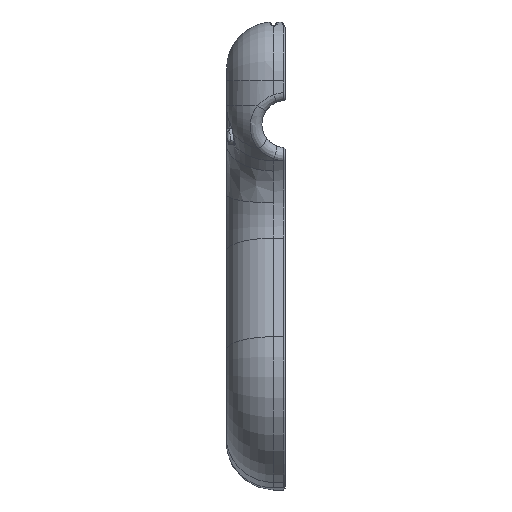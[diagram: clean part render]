
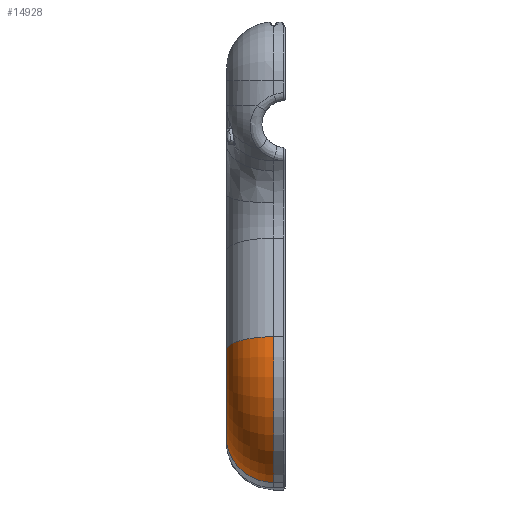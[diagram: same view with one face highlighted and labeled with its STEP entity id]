
A CAD part, left-side view. The second image highlights one B-rep face of the part: STEP entity #14928.
In plain terms, the highlighted toroidal (fillet/blend) face has major radius 18 mm and minor radius 12 mm.
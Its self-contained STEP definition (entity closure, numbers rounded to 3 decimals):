
#3864 = CYLINDRICAL_SURFACE('',#3865,30.);
#3865 = AXIS2_PLACEMENT_3D('',#3866,#3867,#3868);
#3866 = CARTESIAN_POINT('',(-25.893,-15.,-79.431));
#3867 = DIRECTION('',(0.,1.,0.));
#3868 = DIRECTION('',(-0.276,0.,-0.961));
#8954 = VERTEX_POINT('',#8955);
#8955 = CARTESIAN_POINT('',(-34.162,3.,-108.269));
#8992 = CYLINDRICAL_SURFACE('',#8993,12.);
#8993 = AXIS2_PLACEMENT_3D('',#8994,#8995,#8996);
#8994 = CARTESIAN_POINT('',(-26.048,3.,-98.112));
#8995 = DIRECTION('',(-0.961,0.,0.276));
#8996 = DIRECTION('',(-0.276,0.,-0.961));
#9010 = VERTEX_POINT('',#9011);
#9011 = CARTESIAN_POINT('',(-54.731,3.,-71.162));
#9032 = EDGE_CURVE('',#8954,#9010,#9033,.T.);
#9033 = SURFACE_CURVE('',#9034,(#9039,#9046),.PCURVE_S1.);
#9034 = CIRCLE('',#9035,30.);
#9035 = AXIS2_PLACEMENT_3D('',#9036,#9037,#9038);
#9036 = CARTESIAN_POINT('',(-25.893,3.,-79.431));
#9037 = DIRECTION('',(0.,1.,0.));
#9038 = DIRECTION('',(-0.276,0.,-0.961));
#9039 = PCURVE('',#3864,#9040);
#9040 = DEFINITIONAL_REPRESENTATION('',(#9041),#9045);
#9041 = LINE('',#9042,#9043);
#9042 = CARTESIAN_POINT('',(0.,18.));
#9043 = VECTOR('',#9044,1.);
#9044 = DIRECTION('',(1.,0.));
#9045 = ( GEOMETRIC_REPRESENTATION_CONTEXT(2) 
PARAMETRIC_REPRESENTATION_CONTEXT() REPRESENTATION_CONTEXT('2D SPACE',''
  ) );
#9046 = PCURVE('',#9047,#9052);
#9047 = TOROIDAL_SURFACE('',#9048,18.,12.);
#9048 = AXIS2_PLACEMENT_3D('',#9049,#9050,#9051);
#9049 = CARTESIAN_POINT('',(-25.893,3.,-79.431));
#9050 = DIRECTION('',(0.,1.,0.));
#9051 = DIRECTION('',(-0.276,0.,-0.961));
#9052 = DEFINITIONAL_REPRESENTATION('',(#9053),#9057);
#9053 = LINE('',#9054,#9055);
#9054 = CARTESIAN_POINT('',(0.,0.));
#9055 = VECTOR('',#9056,1.);
#9056 = DIRECTION('',(1.,0.));
#9057 = ( GEOMETRIC_REPRESENTATION_CONTEXT(2) 
PARAMETRIC_REPRESENTATION_CONTEXT() REPRESENTATION_CONTEXT('2D SPACE',''
  ) );
#9101 = CYLINDRICAL_SURFACE('',#9102,12.);
#9102 = AXIS2_PLACEMENT_3D('',#9103,#9104,#9105);
#9103 = CARTESIAN_POINT('',(-43.196,3.,-74.47));
#9104 = DIRECTION('',(0.276,0.,0.961));
#9105 = DIRECTION('',(-0.961,0.,0.276));
#14800 = PLANE('',#14801);
#14801 = AXIS2_PLACEMENT_3D('',#14802,#14803,#14804);
#14802 = CARTESIAN_POINT('',(10.936,15.,-32.273));
#14803 = DIRECTION('',(0.,1.,0.));
#14804 = DIRECTION('',(0.,0.,1.));
#14886 = VERTEX_POINT('',#14887);
#14887 = CARTESIAN_POINT('',(-30.855,15.,-96.734));
#14908 = EDGE_CURVE('',#8954,#14886,#14909,.T.);
#14909 = SURFACE_CURVE('',#14910,(#14915,#14921),.PCURVE_S1.);
#14910 = CIRCLE('',#14911,12.);
#14911 = AXIS2_PLACEMENT_3D('',#14912,#14913,#14914);
#14912 = CARTESIAN_POINT('',(-30.855,3.,-96.734));
#14913 = DIRECTION('',(0.961,0.,-0.276));
#14914 = DIRECTION('',(-0.276,0.,-0.961));
#14915 = PCURVE('',#8992,#14916);
#14916 = DEFINITIONAL_REPRESENTATION('',(#14917),#14920);
#14917 = B_SPLINE_CURVE_WITH_KNOTS('',1,(#14918,#14919),.UNSPECIFIED.,
  .F.,.F.,(2,2),(0.,1.571),.PIECEWISE_BEZIER_KNOTS.);
#14918 = CARTESIAN_POINT('',(0.,5.));
#14919 = CARTESIAN_POINT('',(-1.571,5.));
#14920 = ( GEOMETRIC_REPRESENTATION_CONTEXT(2) 
PARAMETRIC_REPRESENTATION_CONTEXT() REPRESENTATION_CONTEXT('2D SPACE',''
  ) );
#14921 = PCURVE('',#9047,#14922);
#14922 = DEFINITIONAL_REPRESENTATION('',(#14923),#14926);
#14923 = B_SPLINE_CURVE_WITH_KNOTS('',1,(#14924,#14925),.UNSPECIFIED.,
  .F.,.F.,(2,2),(0.,1.571),.PIECEWISE_BEZIER_KNOTS.);
#14924 = CARTESIAN_POINT('',(0.,0.));
#14925 = CARTESIAN_POINT('',(0.,1.571));
#14926 = ( GEOMETRIC_REPRESENTATION_CONTEXT(2) 
PARAMETRIC_REPRESENTATION_CONTEXT() REPRESENTATION_CONTEXT('2D SPACE',''
  ) );
#14928 = ADVANCED_FACE('',(#14929),#9047,.T.);
#14929 = FACE_BOUND('',#14930,.T.);
#14930 = EDGE_LOOP('',(#14931,#14932,#14933,#14955));
#14931 = ORIENTED_EDGE('',*,*,#14908,.F.);
#14932 = ORIENTED_EDGE('',*,*,#9032,.T.);
#14933 = ORIENTED_EDGE('',*,*,#14934,.T.);
#14934 = EDGE_CURVE('',#9010,#14935,#14937,.T.);
#14935 = VERTEX_POINT('',#14936);
#14936 = CARTESIAN_POINT('',(-43.196,15.,-74.47));
#14937 = SURFACE_CURVE('',#14938,(#14943,#14949),.PCURVE_S1.);
#14938 = CIRCLE('',#14939,12.);
#14939 = AXIS2_PLACEMENT_3D('',#14940,#14941,#14942);
#14940 = CARTESIAN_POINT('',(-43.196,3.,-74.47));
#14941 = DIRECTION('',(-0.276,0.,-0.961));
#14942 = DIRECTION('',(-0.961,0.,0.276));
#14943 = PCURVE('',#9047,#14944);
#14944 = DEFINITIONAL_REPRESENTATION('',(#14945),#14948);
#14945 = B_SPLINE_CURVE_WITH_KNOTS('',1,(#14946,#14947),.UNSPECIFIED.,
  .F.,.F.,(2,2),(0.,1.571),.PIECEWISE_BEZIER_KNOTS.);
#14946 = CARTESIAN_POINT('',(1.571,0.));
#14947 = CARTESIAN_POINT('',(1.571,1.571));
#14948 = ( GEOMETRIC_REPRESENTATION_CONTEXT(2) 
PARAMETRIC_REPRESENTATION_CONTEXT() REPRESENTATION_CONTEXT('2D SPACE',''
  ) );
#14949 = PCURVE('',#9101,#14950);
#14950 = DEFINITIONAL_REPRESENTATION('',(#14951),#14954);
#14951 = B_SPLINE_CURVE_WITH_KNOTS('',1,(#14952,#14953),.UNSPECIFIED.,
  .F.,.F.,(2,2),(0.,1.571),.PIECEWISE_BEZIER_KNOTS.);
#14952 = CARTESIAN_POINT('',(0.,0.));
#14953 = CARTESIAN_POINT('',(-1.571,0.));
#14954 = ( GEOMETRIC_REPRESENTATION_CONTEXT(2) 
PARAMETRIC_REPRESENTATION_CONTEXT() REPRESENTATION_CONTEXT('2D SPACE',''
  ) );
#14955 = ORIENTED_EDGE('',*,*,#14956,.F.);
#14956 = EDGE_CURVE('',#14886,#14935,#14957,.T.);
#14957 = SURFACE_CURVE('',#14958,(#14963,#14970),.PCURVE_S1.);
#14958 = CIRCLE('',#14959,18.);
#14959 = AXIS2_PLACEMENT_3D('',#14960,#14961,#14962);
#14960 = CARTESIAN_POINT('',(-25.893,15.,-79.431));
#14961 = DIRECTION('',(0.,1.,0.));
#14962 = DIRECTION('',(-0.276,0.,-0.961));
#14963 = PCURVE('',#9047,#14964);
#14964 = DEFINITIONAL_REPRESENTATION('',(#14965),#14969);
#14965 = LINE('',#14966,#14967);
#14966 = CARTESIAN_POINT('',(0.,1.571));
#14967 = VECTOR('',#14968,1.);
#14968 = DIRECTION('',(1.,0.));
#14969 = ( GEOMETRIC_REPRESENTATION_CONTEXT(2) 
PARAMETRIC_REPRESENTATION_CONTEXT() REPRESENTATION_CONTEXT('2D SPACE',''
  ) );
#14970 = PCURVE('',#14800,#14971);
#14971 = DEFINITIONAL_REPRESENTATION('',(#14972),#14976);
#14972 = CIRCLE('',#14973,18.);
#14973 = AXIS2_PLACEMENT_2D('',#14974,#14975);
#14974 = CARTESIAN_POINT('',(-47.158,-36.829));
#14975 = DIRECTION('',(-0.961,-0.276));
#14976 = ( GEOMETRIC_REPRESENTATION_CONTEXT(2) 
PARAMETRIC_REPRESENTATION_CONTEXT() REPRESENTATION_CONTEXT('2D SPACE',''
  ) );
